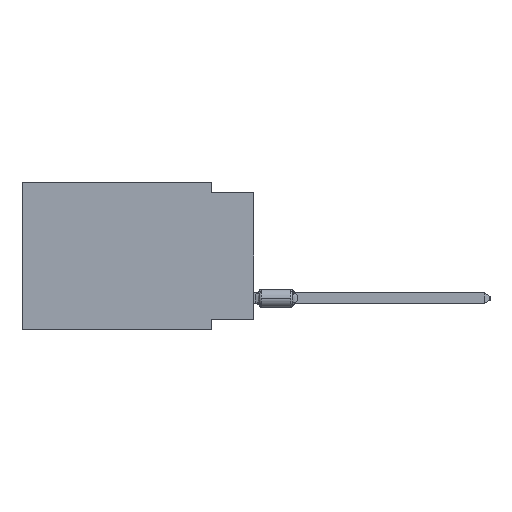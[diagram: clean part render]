
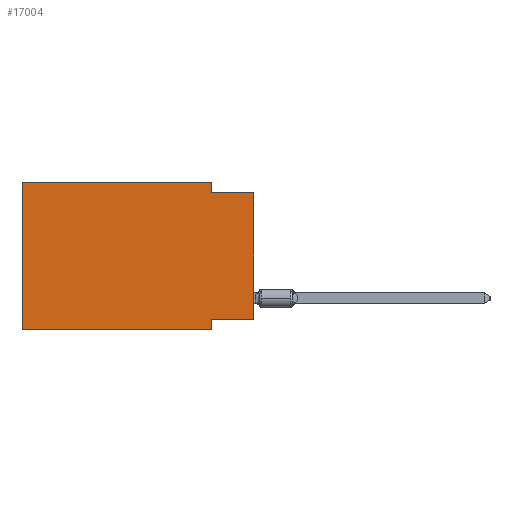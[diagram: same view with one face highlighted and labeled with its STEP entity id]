
A CAD part, left-side view. The second image highlights one B-rep face of the part: STEP entity #17004.
In plain terms, the highlighted planar face has unit normal (-1, 0, 0).
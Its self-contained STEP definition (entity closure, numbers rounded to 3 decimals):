
#70 = LINE ( 'NONE', #10236, #6396 ) ;
#349 = CARTESIAN_POINT ( 'NONE',  ( 0., 0., -8.255 ) ) ;
#1726 = VECTOR ( 'NONE', #11221, 1000. ) ;
#1787 = CARTESIAN_POINT ( 'NONE',  ( 0., 0., -0.635 ) ) ;
#1798 = CARTESIAN_POINT ( 'NONE',  ( 0., 2.54, -8.89 ) ) ;
#2315 = CARTESIAN_POINT ( 'NONE',  ( 0., 2.54, -8.255 ) ) ;
#2589 = EDGE_CURVE ( 'NONE', #7585, #21050, #32426, .T. ) ;
#2663 = DIRECTION ( 'NONE',  ( 1., 0., 0. ) ) ;
#3712 = CARTESIAN_POINT ( 'NONE',  ( 0., 0., -8.255 ) ) ;
#4020 = CARTESIAN_POINT ( 'NONE',  ( 0., 2.54, 0. ) ) ;
#4425 = DIRECTION ( 'NONE',  ( 0., 0., -1. ) ) ;
#5338 = ORIENTED_EDGE ( 'NONE', *, *, #8489, .F. ) ;
#5611 = ORIENTED_EDGE ( 'NONE', *, *, #31196, .F. ) ;
#6396 = VECTOR ( 'NONE', #15398, 1000. ) ;
#6772 = DIRECTION ( 'NONE',  ( 0., -1., 0. ) ) ;
#7585 = VERTEX_POINT ( 'NONE', #4020 ) ;
#8489 = EDGE_CURVE ( 'NONE', #32709, #28493, #9424, .T. ) ;
#9424 = LINE ( 'NONE', #3712, #1726 ) ;
#9987 = EDGE_CURVE ( 'NONE', #32709, #18920, #13417, .T. ) ;
#10178 = VECTOR ( 'NONE', #17556, 1000. ) ;
#10236 = CARTESIAN_POINT ( 'NONE',  ( 0., 13.97, 0. ) ) ;
#10409 = CARTESIAN_POINT ( 'NONE',  ( 0., 2.54, -8.89 ) ) ;
#11221 = DIRECTION ( 'NONE',  ( 0., 1., 0. ) ) ;
#12347 = AXIS2_PLACEMENT_3D ( 'NONE', #13493, #2663, #18001 ) ;
#13335 = CARTESIAN_POINT ( 'NONE',  ( 0., 0., -0.635 ) ) ;
#13417 = LINE ( 'NONE', #18430, #15315 ) ;
#13493 = CARTESIAN_POINT ( 'NONE',  ( 0., 13.97, 0. ) ) ;
#15117 = VECTOR ( 'NONE', #25445, 1000. ) ;
#15315 = VECTOR ( 'NONE', #23614, 1000. ) ;
#15398 = DIRECTION ( 'NONE',  ( 0., 0., 1. ) ) ;
#16350 = EDGE_CURVE ( 'NONE', #21058, #21239, #20402, .T. ) ;
#17004 = ADVANCED_FACE ( 'NONE', ( #26187 ), #30682, .F. ) ;
#17556 = DIRECTION ( 'NONE',  ( 0., -1., 0. ) ) ;
#18001 = DIRECTION ( 'NONE',  ( 0., 0., -1. ) ) ;
#18197 = CARTESIAN_POINT ( 'NONE',  ( 0., 13.97, 0. ) ) ;
#18430 = CARTESIAN_POINT ( 'NONE',  ( 0., 0., 0. ) ) ;
#18719 = VECTOR ( 'NONE', #20202, 1000. ) ;
#18920 = VERTEX_POINT ( 'NONE', #1787 ) ;
#18988 = ORIENTED_EDGE ( 'NONE', *, *, #16350, .T. ) ;
#19588 = CARTESIAN_POINT ( 'NONE',  ( 0., 2.54, 0. ) ) ;
#19628 = CARTESIAN_POINT ( 'NONE',  ( 0., 13.97, 0. ) ) ;
#20202 = DIRECTION ( 'NONE',  ( 0., -1., 0. ) ) ;
#20402 = LINE ( 'NONE', #25264, #10178 ) ;
#20501 = EDGE_CURVE ( 'NONE', #21058, #32655, #70, .T. ) ;
#21050 = VERTEX_POINT ( 'NONE', #28816 ) ;
#21058 = VERTEX_POINT ( 'NONE', #31657 ) ;
#21239 = VERTEX_POINT ( 'NONE', #1798 ) ;
#21825 = VECTOR ( 'NONE', #6772, 1000. ) ;
#22130 = ORIENTED_EDGE ( 'NONE', *, *, #24640, .F. ) ;
#23065 = VECTOR ( 'NONE', #4425, 1000. ) ;
#23112 = LINE ( 'NONE', #10409, #15117 ) ;
#23176 = EDGE_LOOP ( 'NONE', ( #28879, #25261, #25940, #5611, #31295, #18988, #22130, #5338 ) ) ;
#23614 = DIRECTION ( 'NONE',  ( 0., 0., 1. ) ) ;
#24640 = EDGE_CURVE ( 'NONE', #28493, #21239, #23112, .T. ) ;
#25261 = ORIENTED_EDGE ( 'NONE', *, *, #32681, .F. ) ;
#25264 = CARTESIAN_POINT ( 'NONE',  ( 0., 13.97, -8.89 ) ) ;
#25445 = DIRECTION ( 'NONE',  ( 0., 0., -1. ) ) ;
#25940 = ORIENTED_EDGE ( 'NONE', *, *, #2589, .F. ) ;
#26187 = FACE_OUTER_BOUND ( 'NONE', #23176, .T. ) ;
#28203 = LINE ( 'NONE', #13335, #18719 ) ;
#28493 = VERTEX_POINT ( 'NONE', #2315 ) ;
#28816 = CARTESIAN_POINT ( 'NONE',  ( 0., 2.54, -0.635 ) ) ;
#28879 = ORIENTED_EDGE ( 'NONE', *, *, #9987, .T. ) ;
#30682 = PLANE ( 'NONE',  #12347 ) ;
#31196 = EDGE_CURVE ( 'NONE', #32655, #7585, #32150, .T. ) ;
#31295 = ORIENTED_EDGE ( 'NONE', *, *, #20501, .F. ) ;
#31657 = CARTESIAN_POINT ( 'NONE',  ( 0., 13.97, -8.89 ) ) ;
#32150 = LINE ( 'NONE', #19628, #21825 ) ;
#32426 = LINE ( 'NONE', #19588, #23065 ) ;
#32655 = VERTEX_POINT ( 'NONE', #18197 ) ;
#32681 = EDGE_CURVE ( 'NONE', #21050, #18920, #28203, .T. ) ;
#32709 = VERTEX_POINT ( 'NONE', #349 ) ;
